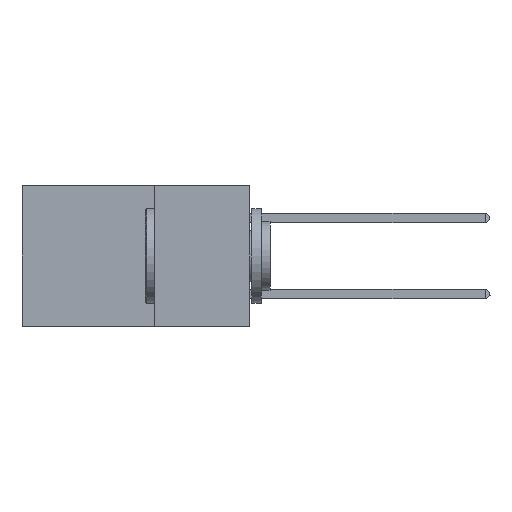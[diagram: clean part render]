
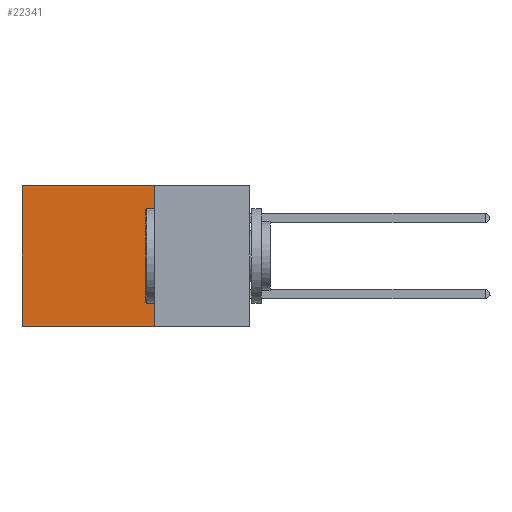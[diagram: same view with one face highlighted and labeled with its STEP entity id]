
A CAD part, left-side view. The second image highlights one B-rep face of the part: STEP entity #22341.
In plain terms, the highlighted planar face has unit normal (-1, 0, 0).
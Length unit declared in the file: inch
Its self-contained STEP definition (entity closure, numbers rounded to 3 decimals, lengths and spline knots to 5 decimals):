
#1862 = AXIS2_PLACEMENT_3D ( 'NONE', #44998, #35641, #42082 ) ;
#2980 = LINE ( 'NONE', #5501, #14480 ) ;
#3960 = ORIENTED_EDGE ( 'NONE', *, *, #41069, .T. ) ;
#5156 = VECTOR ( 'NONE', #40648, 39.37008 ) ;
#5501 = CARTESIAN_POINT ( 'NONE',  ( 0.2875, 0.6, 0. ) ) ;
#5510 = EDGE_CURVE ( 'NONE', #38167, #36763, #37313, .T. ) ;
#6762 = VERTEX_POINT ( 'NONE', #9750 ) ;
#8935 = ORIENTED_EDGE ( 'NONE', *, *, #5510, .F. ) ;
#9627 = CARTESIAN_POINT ( 'NONE',  ( 0.2875, 0.6, -0.37 ) ) ;
#9750 = CARTESIAN_POINT ( 'NONE',  ( 0.2875, 0.6, 0. ) ) ;
#9920 = PLANE ( 'NONE',  #1862 ) ;
#11276 = LINE ( 'NONE', #16278, #39218 ) ;
#13136 = VERTEX_POINT ( 'NONE', #23098 ) ;
#14480 = VECTOR ( 'NONE', #39777, 39.37008 ) ;
#16278 = CARTESIAN_POINT ( 'NONE',  ( 0.2875, 0.25, 0. ) ) ;
#22341 = ADVANCED_FACE ( 'NONE', ( #33025 ), #9920, .F. ) ;
#23098 = CARTESIAN_POINT ( 'NONE',  ( 0.2875, 0.25, 0. ) ) ;
#23887 = CARTESIAN_POINT ( 'NONE',  ( 0.2875, 0.25, -0.37 ) ) ;
#25919 = LINE ( 'NONE', #29949, #5156 ) ;
#29217 = EDGE_LOOP ( 'NONE', ( #42759, #8935, #33637, #3960 ) ) ;
#29949 = CARTESIAN_POINT ( 'NONE',  ( 0.2875, 0.25, 0. ) ) ;
#32803 = DIRECTION ( 'NONE',  ( 0., 1., 0. ) ) ;
#33025 = FACE_OUTER_BOUND ( 'NONE', #29217, .T. ) ;
#33637 = ORIENTED_EDGE ( 'NONE', *, *, #37283, .F. ) ;
#35641 = DIRECTION ( 'NONE',  ( 1., 0., 0. ) ) ;
#36763 = VERTEX_POINT ( 'NONE', #9627 ) ;
#37283 = EDGE_CURVE ( 'NONE', #13136, #38167, #25919, .T. ) ;
#37313 = LINE ( 'NONE', #39960, #38407 ) ;
#38167 = VERTEX_POINT ( 'NONE', #23887 ) ;
#38407 = VECTOR ( 'NONE', #32803, 39.37008 ) ;
#39218 = VECTOR ( 'NONE', #44272, 39.37008 ) ;
#39777 = DIRECTION ( 'NONE',  ( 0., 0., -1. ) ) ;
#39960 = CARTESIAN_POINT ( 'NONE',  ( 0.2875, 0.25, -0.37 ) ) ;
#40648 = DIRECTION ( 'NONE',  ( 0., 0., -1. ) ) ;
#41069 = EDGE_CURVE ( 'NONE', #13136, #6762, #11276, .T. ) ;
#42082 = DIRECTION ( 'NONE',  ( 0., 0., -1. ) ) ;
#42441 = EDGE_CURVE ( 'NONE', #6762, #36763, #2980, .T. ) ;
#42759 = ORIENTED_EDGE ( 'NONE', *, *, #42441, .T. ) ;
#44272 = DIRECTION ( 'NONE',  ( 0., 1., 0. ) ) ;
#44998 = CARTESIAN_POINT ( 'NONE',  ( 0.2875, 0.25, 0. ) ) ;
